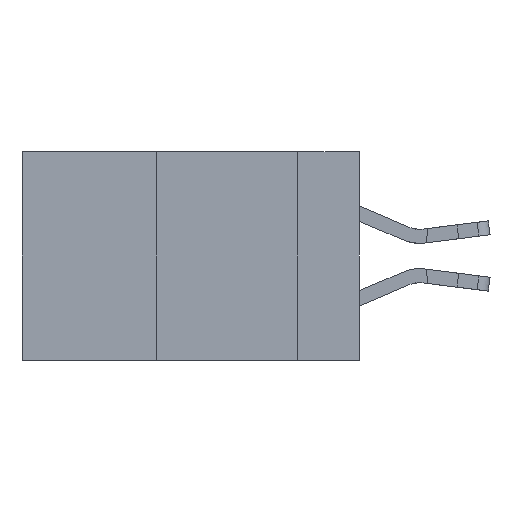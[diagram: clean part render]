
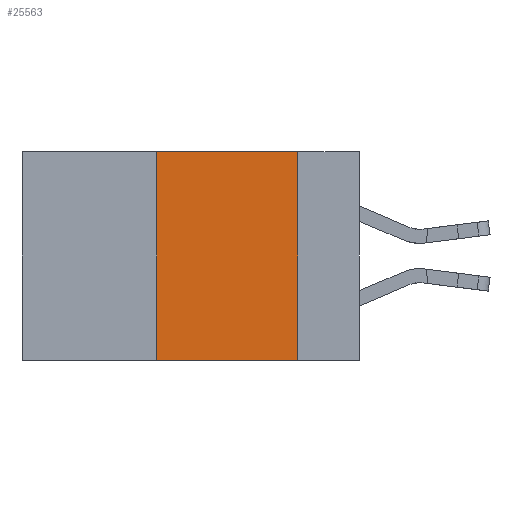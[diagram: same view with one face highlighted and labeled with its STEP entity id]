
A CAD part, left-side view. The second image highlights one B-rep face of the part: STEP entity #25563.
In plain terms, the highlighted planar face has unit normal (-1, 0, 0).
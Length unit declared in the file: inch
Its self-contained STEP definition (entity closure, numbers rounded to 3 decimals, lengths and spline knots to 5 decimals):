
#713 = CARTESIAN_POINT ( 'NONE',  ( 0., 0.11, 0. ) ) ;
#865 = VERTEX_POINT ( 'NONE', #30115 ) ;
#1119 = LINE ( 'NONE', #30015, #18970 ) ;
#2120 = ORIENTED_EDGE ( 'NONE', *, *, #22288, .F. ) ;
#2933 = VECTOR ( 'NONE', #16219, 39.37008 ) ;
#3285 = VERTEX_POINT ( 'NONE', #9758 ) ;
#3959 = DIRECTION ( 'NONE',  ( 0., 0., -1. ) ) ;
#6250 = VECTOR ( 'NONE', #3959, 39.37008 ) ;
#6394 = ORIENTED_EDGE ( 'NONE', *, *, #8548, .F. ) ;
#6429 = FACE_OUTER_BOUND ( 'NONE', #16990, .T. ) ;
#8548 = EDGE_CURVE ( 'NONE', #865, #3285, #1119, .T. ) ;
#9758 = CARTESIAN_POINT ( 'NONE',  ( 0., 0.36, 0. ) ) ;
#10021 = DIRECTION ( 'NONE',  ( 1., 0., 0. ) ) ;
#10096 = VERTEX_POINT ( 'NONE', #713 ) ;
#11282 = VECTOR ( 'NONE', #29252, 39.37008 ) ;
#15398 = CARTESIAN_POINT ( 'NONE',  ( 0., 0.11, -0.37 ) ) ;
#16219 = DIRECTION ( 'NONE',  ( 0., -1., 0. ) ) ;
#16990 = EDGE_LOOP ( 'NONE', ( #29150, #2120, #6394, #33000 ) ) ;
#17685 = CARTESIAN_POINT ( 'NONE',  ( 0., 0.11, 0. ) ) ;
#18636 = CARTESIAN_POINT ( 'NONE',  ( 0., 0.6, -0.37 ) ) ;
#18970 = VECTOR ( 'NONE', #32693, 39.37008 ) ;
#22288 = EDGE_CURVE ( 'NONE', #3285, #10096, #35458, .T. ) ;
#23823 = PLANE ( 'NONE',  #31333 ) ;
#24810 = EDGE_CURVE ( 'NONE', #865, #28922, #30711, .T. ) ;
#25563 = ADVANCED_FACE ( 'NONE', ( #6429 ), #23823, .F. ) ;
#28922 = VERTEX_POINT ( 'NONE', #15398 ) ;
#29150 = ORIENTED_EDGE ( 'NONE', *, *, #34185, .F. ) ;
#29210 = LINE ( 'NONE', #17685, #6250 ) ;
#29252 = DIRECTION ( 'NONE',  ( 0., -1., 0. ) ) ;
#29449 = DIRECTION ( 'NONE',  ( 0., 0., -1. ) ) ;
#30015 = CARTESIAN_POINT ( 'NONE',  ( 0., 0.36, 0. ) ) ;
#30115 = CARTESIAN_POINT ( 'NONE',  ( 0., 0.36, -0.37 ) ) ;
#30711 = LINE ( 'NONE', #18636, #11282 ) ;
#31333 = AXIS2_PLACEMENT_3D ( 'NONE', #32100, #10021, #29449 ) ;
#32100 = CARTESIAN_POINT ( 'NONE',  ( 0., 0.6, 0. ) ) ;
#32693 = DIRECTION ( 'NONE',  ( 0., 0., 1. ) ) ;
#32751 = CARTESIAN_POINT ( 'NONE',  ( 0., 0.6, 0. ) ) ;
#33000 = ORIENTED_EDGE ( 'NONE', *, *, #24810, .T. ) ;
#34185 = EDGE_CURVE ( 'NONE', #10096, #28922, #29210, .T. ) ;
#35458 = LINE ( 'NONE', #32751, #2933 ) ;
